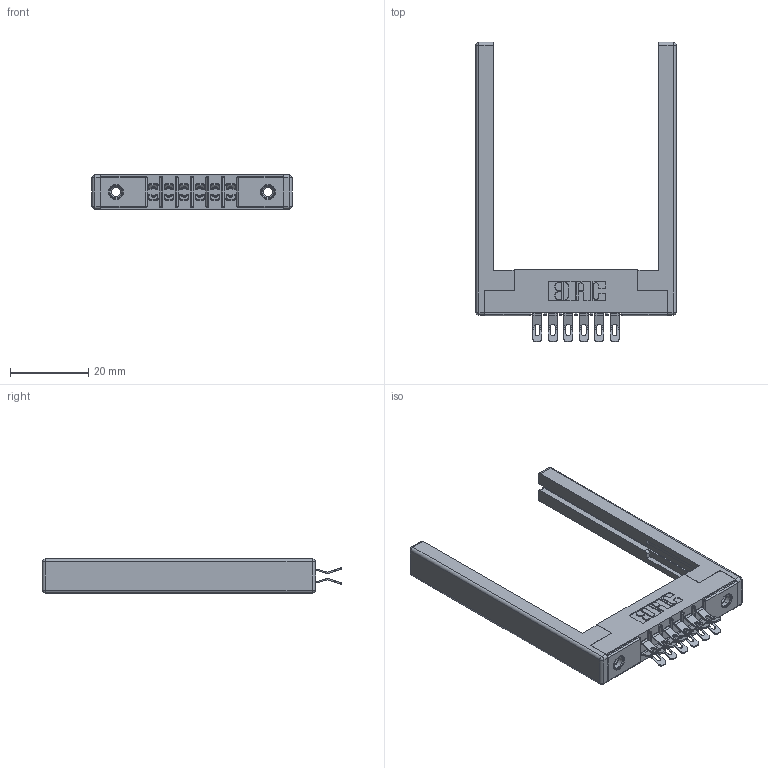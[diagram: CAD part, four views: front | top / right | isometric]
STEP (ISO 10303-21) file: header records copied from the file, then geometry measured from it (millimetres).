
FILE_DESCRIPTION (( 'STEP AP203' ), '1' );
FILE_NAME ('315-012-555-268.STEP', '2019-09-10T13:22:21', ( '' ), ( '' ), 'SwSTEP 2.0', 'SolidWorks 2016', '' );
FILE_SCHEMA (( 'CONFIG_CONTROL_DESIGN' ));
Length unit declared in the file: inch
Products named in the file (5): 305 Part_.156 Dia; 315-012-555-268; 305-290-001_555; 307-220-068; 345-250-001_345-250-001-102
Assembly tree (17 placements, depth 2):
  315-012-555-268
    305 Part_.156 Dia
    305-290-001_555  x12
    345-250-001_345-250-001-102  x2
    307-220-068  x2
Bounding box: 51.21 x 76.71 x 8.71 mm (x, y, z)
Volume: 7848.7 mm3; surface area: 9467.9 mm2
Topology: 17 solids, 17 shells, 1062 faces, 3076 edges, 1996 vertices
Faces by surface type: plane 540, cylinder 474, sphere 32, cone 12, torus 4
Entity records: 14262 total; most frequent: CARTESIAN_POINT 2351, DIRECTION 2317, ORIENTED_EDGE 2310, EDGE_CURVE 1155, VECTOR 865, LINE 865, VERTEX_POINT 744, AXIS2_PLACEMENT_3D 726
